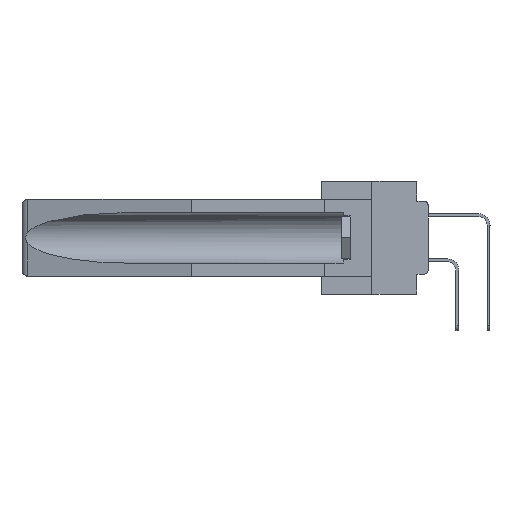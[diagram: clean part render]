
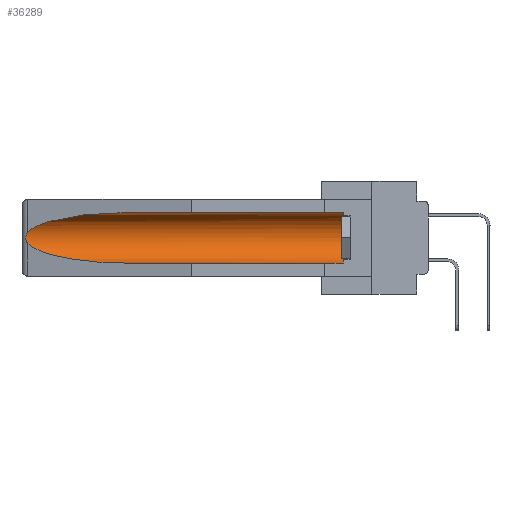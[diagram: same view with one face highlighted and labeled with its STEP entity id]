
A CAD part, left-side view. The second image highlights one B-rep face of the part: STEP entity #36289.
In plain terms, the highlighted cylindrical face has radius 2.857 mm (diameter 5.715 mm), a partial arc.
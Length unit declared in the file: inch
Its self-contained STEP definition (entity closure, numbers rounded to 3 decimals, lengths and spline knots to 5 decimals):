
#328 = EDGE_LOOP ( 'NONE', ( #38837, #1381, #27341, #28678, #23025, #4525 ) ) ;
#638 = LINE ( 'NONE', #2166, #29353 ) ;
#658 = CARTESIAN_POINT ( 'NONE',  ( 0.155, -0.30754, -0.1715 ) ) ;
#1381 = ORIENTED_EDGE ( 'NONE', *, *, #11040, .T. ) ;
#2166 = CARTESIAN_POINT ( 'NONE',  ( 0.155, -0.30754, -0.284 ) ) ;
#2253 = CARTESIAN_POINT ( 'NONE',  ( 0.26537, 1.52718, -0.14972 ) ) ;
#3189 = CARTESIAN_POINT ( 'NONE',  ( 0.21114, 1.30732, -0.284 ) ) ;
#4525 = ORIENTED_EDGE ( 'NONE', *, *, #37808, .T. ) ;
#5234 = CARTESIAN_POINT ( 'NONE',  ( 0.26537, 1.52718, -0.19328 ) ) ;
#5801 = DIRECTION ( 'NONE',  ( 0., 1., 0. ) ) ;
#6491 = CARTESIAN_POINT ( 'NONE',  ( 0.21114, 1.30732, -0.059 ) ) ;
#7300 = CARTESIAN_POINT ( 'NONE',  ( 0.155, 0.126, -0.284 ) ) ;
#8061 = CIRCLE ( 'NONE', #24633, 0.1125 ) ;
#8433 = CARTESIAN_POINT ( 'NONE',  ( 0.155, -0.30754, -0.059 ) ) ;
#8499 = VERTEX_POINT ( 'NONE', #28430 ) ;
#8649 = CARTESIAN_POINT ( 'NONE',  ( 0.2673, 1.53269, -0.17917 ) ) ;
#9599 = CARTESIAN_POINT ( 'NONE',  ( 0.25451, 1.48313, -0.24835 ) ) ;
#9692 = CYLINDRICAL_SURFACE ( 'NONE', #32996, 0.1125 ) ;
#10475 = CARTESIAN_POINT ( 'NONE',  ( 0.155, 0.126, -0.059 ) ) ;
#10574 = EDGE_CURVE ( 'NONE', #36704, #13807, #8061, .T. ) ;
#11040 = EDGE_CURVE ( 'NONE', #24187, #8499, #29649, .T. ) ;
#11268 = CARTESIAN_POINT ( 'NONE',  ( 0.26597, 1.52961, -0.15275 ) ) ;
#12190 = DIRECTION ( 'NONE',  ( 0., 0., 1. ) ) ;
#12460 = EDGE_CURVE ( 'NONE', #8499, #33971, #37644, .T. ) ;
#12699 = CARTESIAN_POINT ( 'NONE',  ( 0.26537, 1.52718, -0.14972 ) ) ;
#13314 = VECTOR ( 'NONE', #5801, 39.37008 ) ;
#13807 = VERTEX_POINT ( 'NONE', #10475 ) ;
#14275 = CARTESIAN_POINT ( 'NONE',  ( 0.26654, 1.53092, -0.15636 ) ) ;
#14856 = VERTEX_POINT ( 'NONE', #27511 ) ;
#15657 = CARTESIAN_POINT ( 'NONE',  ( 0.155, 1.07973, -0.284 ) ) ;
#17237 = CARTESIAN_POINT ( 'NONE',  ( 0.26597, 1.5296, -0.19026 ) ) ;
#17365 = CARTESIAN_POINT ( 'NONE',  ( 0.2675, 1.53308, -0.17534 ) ) ;
#17498 = CARTESIAN_POINT ( 'NONE',  ( 0.2673, 1.5327, -0.16383 ) ) ;
#18703 = DIRECTION ( 'NONE',  ( 0., 1., 0. ) ) ;
#18816 = CARTESIAN_POINT ( 'NONE',  ( 0.155, 1.07973, -0.284 ) ) ;
#19530 = EDGE_CURVE ( 'NONE', #14856, #24187, #23609, .T. ) ;
#23025 = ORIENTED_EDGE ( 'NONE', *, *, #10574, .T. ) ;
#23228 = CARTESIAN_POINT ( 'NONE',  ( 0.2675, 1.53308, -0.16763 ) ) ;
#23609 =( BOUNDED_CURVE ( )  B_SPLINE_CURVE ( 3, ( #24624, #6491, #36868, #30427 ),
 .UNSPECIFIED., .F., .F. ) 
 B_SPLINE_CURVE_WITH_KNOTS ( ( 4, 4 ),
 ( 4.71239, 6.08839 ),
 .UNSPECIFIED. ) 
 CURVE ( )  GEOMETRIC_REPRESENTATION_ITEM ( )  RATIONAL_B_SPLINE_CURVE ( ( 1., 0.848, 0.848, 1. ) ) 
 REPRESENTATION_ITEM ( '' )  );
#24187 = VERTEX_POINT ( 'NONE', #12699 ) ;
#24624 = CARTESIAN_POINT ( 'NONE',  ( 0.155, 1.07973, -0.059 ) ) ;
#24633 = AXIS2_PLACEMENT_3D ( 'NONE', #32394, #26462, #38311 ) ;
#25571 = LINE ( 'NONE', #8433, #13314 ) ;
#26068 = DIRECTION ( 'NONE',  ( 0., 1., 0. ) ) ;
#26462 = DIRECTION ( 'NONE',  ( 0., -1., 0. ) ) ;
#27341 = ORIENTED_EDGE ( 'NONE', *, *, #12460, .T. ) ;
#27511 = CARTESIAN_POINT ( 'NONE',  ( 0.155, 1.07973, -0.059 ) ) ;
#28430 = CARTESIAN_POINT ( 'NONE',  ( 0.26537, 1.52718, -0.19328 ) ) ;
#28678 = ORIENTED_EDGE ( 'NONE', *, *, #37686, .F. ) ;
#29042 = FACE_OUTER_BOUND ( 'NONE', #328, .T. ) ;
#29353 = VECTOR ( 'NONE', #26068, 39.37008 ) ;
#29445 = CARTESIAN_POINT ( 'NONE',  ( 0.26655, 1.53094, -0.18657 ) ) ;
#29649 = B_SPLINE_CURVE_WITH_KNOTS ( 'NONE', 3,
 ( #2253, #11268, #14275, #17498, #23228, #17365, #8649, #29445, #17237, #5234 ),
 .UNSPECIFIED., .F., .F.,
 ( 4, 2, 2, 2, 4 ),
 ( 0., 0.00029, 0.00058, 0.00087, 0.00117 ),
 .UNSPECIFIED. ) ;
#30427 = CARTESIAN_POINT ( 'NONE',  ( 0.26537, 1.52718, -0.14972 ) ) ;
#32394 = CARTESIAN_POINT ( 'NONE',  ( 0.155, 0.126, -0.1715 ) ) ;
#32996 = AXIS2_PLACEMENT_3D ( 'NONE', #658, #18703, #12190 ) ;
#33971 = VERTEX_POINT ( 'NONE', #18816 ) ;
#36289 = ADVANCED_FACE ( 'NONE', ( #29042 ), #9692, .F. ) ;
#36580 = CARTESIAN_POINT ( 'NONE',  ( 0.26537, 1.52718, -0.19328 ) ) ;
#36704 = VERTEX_POINT ( 'NONE', #7300 ) ;
#36868 = CARTESIAN_POINT ( 'NONE',  ( 0.25451, 1.48313, -0.09465 ) ) ;
#37644 =( BOUNDED_CURVE ( )  B_SPLINE_CURVE ( 3, ( #36580, #9599, #3189, #15657 ),
 .UNSPECIFIED., .F., .T. ) 
 B_SPLINE_CURVE_WITH_KNOTS ( ( 4, 4 ),
 ( 0.1948, 1.5708 ),
 .UNSPECIFIED. ) 
 CURVE ( )  GEOMETRIC_REPRESENTATION_ITEM ( )  RATIONAL_B_SPLINE_CURVE ( ( 1., 0.848, 0.848, 1. ) ) 
 REPRESENTATION_ITEM ( '' )  );
#37686 = EDGE_CURVE ( 'NONE', #36704, #33971, #638, .T. ) ;
#37808 = EDGE_CURVE ( 'NONE', #13807, #14856, #25571, .T. ) ;
#38311 = DIRECTION ( 'NONE',  ( 0., 0., 1. ) ) ;
#38837 = ORIENTED_EDGE ( 'NONE', *, *, #19530, .T. ) ;
